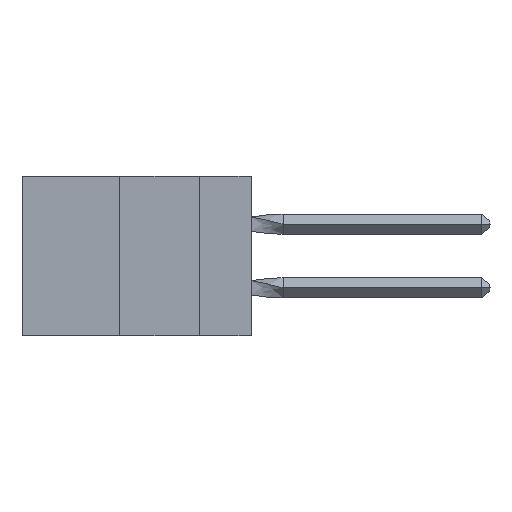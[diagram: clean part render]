
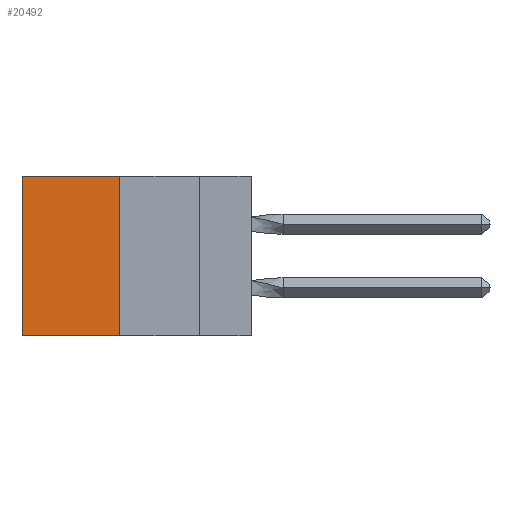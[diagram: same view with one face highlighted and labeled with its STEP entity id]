
A CAD part, left-side view. The second image highlights one B-rep face of the part: STEP entity #20492.
In plain terms, the highlighted planar face has unit normal (-1, 0, 0).
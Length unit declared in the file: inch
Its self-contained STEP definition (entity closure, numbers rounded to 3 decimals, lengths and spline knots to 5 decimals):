
#688 = DIRECTION ( 'NONE',  ( 0., 0., -1. ) ) ;
#837 = CARTESIAN_POINT ( 'NONE',  ( 0.305, 0.413, 0. ) ) ;
#2814 = ORIENTED_EDGE ( 'NONE', *, *, #27666, .F. ) ;
#3099 = ORIENTED_EDGE ( 'NONE', *, *, #18312, .F. ) ;
#3617 = ORIENTED_EDGE ( 'NONE', *, *, #22624, .T. ) ;
#4133 = CARTESIAN_POINT ( 'NONE',  ( 0.305, 0.72, -0.5 ) ) ;
#4450 = ORIENTED_EDGE ( 'NONE', *, *, #36258, .T. ) ;
#4706 = EDGE_LOOP ( 'NONE', ( #4450, #2814, #3099, #3617 ) ) ;
#5064 = DIRECTION ( 'NONE',  ( 0., 0., -1. ) ) ;
#5419 = VECTOR ( 'NONE', #6657, 39.37008 ) ;
#6657 = DIRECTION ( 'NONE',  ( 0., 1., 0. ) ) ;
#9349 = VECTOR ( 'NONE', #15501, 39.37008 ) ;
#11834 = VERTEX_POINT ( 'NONE', #35538 ) ;
#12043 = CARTESIAN_POINT ( 'NONE',  ( 0.305, 0.72, -0.5 ) ) ;
#12657 = VECTOR ( 'NONE', #16432, 39.37008 ) ;
#14871 = LINE ( 'NONE', #33615, #12657 ) ;
#15129 = CARTESIAN_POINT ( 'NONE',  ( 0.305, 0.413, -0.5 ) ) ;
#15501 = DIRECTION ( 'NONE',  ( 0., 0., -1. ) ) ;
#16083 = CARTESIAN_POINT ( 'NONE',  ( 0.305, 0.413, -0.5 ) ) ;
#16432 = DIRECTION ( 'NONE',  ( 0., 1., 0. ) ) ;
#17178 = VERTEX_POINT ( 'NONE', #4133 ) ;
#18312 = EDGE_CURVE ( 'NONE', #34288, #36682, #18732, .T. ) ;
#18732 = LINE ( 'NONE', #15129, #9349 ) ;
#18933 = DIRECTION ( 'NONE',  ( 1., 0., 0. ) ) ;
#19683 = CARTESIAN_POINT ( 'NONE',  ( 0.305, 0.413, -0.5 ) ) ;
#20492 = ADVANCED_FACE ( 'NONE', ( #22521 ), #36383, .F. ) ;
#22365 = AXIS2_PLACEMENT_3D ( 'NONE', #16083, #18933, #5064 ) ;
#22521 = FACE_OUTER_BOUND ( 'NONE', #4706, .T. ) ;
#22624 = EDGE_CURVE ( 'NONE', #34288, #11834, #30451, .T. ) ;
#27666 = EDGE_CURVE ( 'NONE', #36682, #17178, #14871, .T. ) ;
#28133 = CARTESIAN_POINT ( 'NONE',  ( 0.305, 0.413, 0. ) ) ;
#30015 = LINE ( 'NONE', #12043, #35461 ) ;
#30451 = LINE ( 'NONE', #837, #5419 ) ;
#33615 = CARTESIAN_POINT ( 'NONE',  ( 0.305, 0.413, -0.5 ) ) ;
#34288 = VERTEX_POINT ( 'NONE', #28133 ) ;
#35461 = VECTOR ( 'NONE', #688, 39.37008 ) ;
#35538 = CARTESIAN_POINT ( 'NONE',  ( 0.305, 0.72, 0. ) ) ;
#36258 = EDGE_CURVE ( 'NONE', #11834, #17178, #30015, .T. ) ;
#36383 = PLANE ( 'NONE',  #22365 ) ;
#36682 = VERTEX_POINT ( 'NONE', #19683 ) ;
